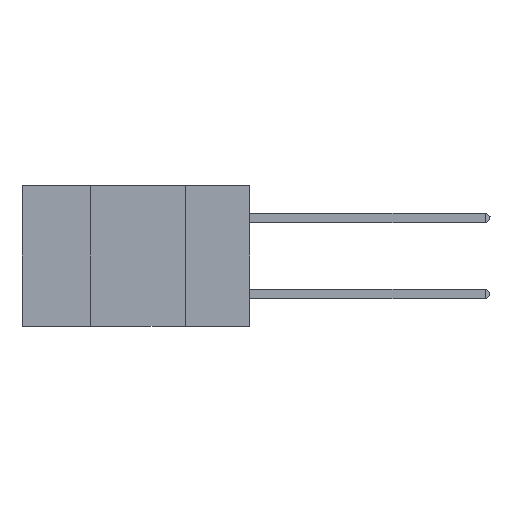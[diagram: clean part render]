
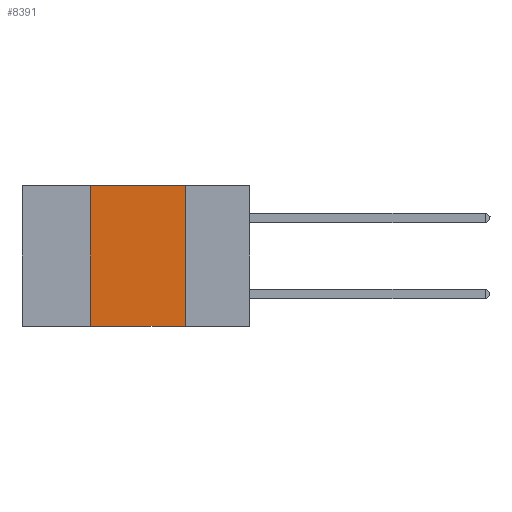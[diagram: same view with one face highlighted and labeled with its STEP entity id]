
A CAD part, left-side view. The second image highlights one B-rep face of the part: STEP entity #8391.
In plain terms, the highlighted planar face has unit normal (-1, 0, 0).
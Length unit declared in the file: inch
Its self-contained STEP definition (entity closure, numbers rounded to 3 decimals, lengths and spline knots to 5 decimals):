
#158 = CARTESIAN_POINT ( 'NONE',  ( 0., 0.42, 0. ) ) ;
#355 = VECTOR ( 'NONE', #10281, 39.37008 ) ;
#591 = EDGE_LOOP ( 'NONE', ( #8766, #2597, #5451, #9386 ) ) ;
#1286 = EDGE_CURVE ( 'NONE', #2280, #1753, #9003, .T. ) ;
#1416 = DIRECTION ( 'NONE',  ( 0., -1., 0. ) ) ;
#1703 = PLANE ( 'NONE',  #7467 ) ;
#1753 = VERTEX_POINT ( 'NONE', #158 ) ;
#2150 = EDGE_CURVE ( 'NONE', #5757, #7885, #3009, .T. ) ;
#2280 = VERTEX_POINT ( 'NONE', #3708 ) ;
#2571 = DIRECTION ( 'NONE',  ( 0., 0., -1. ) ) ;
#2597 = ORIENTED_EDGE ( 'NONE', *, *, #6865, .F. ) ;
#2881 = CARTESIAN_POINT ( 'NONE',  ( 0., 0.17, 0. ) ) ;
#3009 = LINE ( 'NONE', #8593, #3290 ) ;
#3290 = VECTOR ( 'NONE', #4409, 39.37008 ) ;
#3360 = CARTESIAN_POINT ( 'NONE',  ( 0., 0.6, 0. ) ) ;
#3565 = CARTESIAN_POINT ( 'NONE',  ( 0., 0.6, 0. ) ) ;
#3708 = CARTESIAN_POINT ( 'NONE',  ( 0., 0.42, -0.37 ) ) ;
#4179 = EDGE_CURVE ( 'NONE', #2280, #7885, #5869, .T. ) ;
#4409 = DIRECTION ( 'NONE',  ( 0., 0., -1. ) ) ;
#4703 = FACE_OUTER_BOUND ( 'NONE', #591, .T. ) ;
#5310 = VECTOR ( 'NONE', #1416, 39.37008 ) ;
#5451 = ORIENTED_EDGE ( 'NONE', *, *, #1286, .F. ) ;
#5757 = VERTEX_POINT ( 'NONE', #2881 ) ;
#5869 = LINE ( 'NONE', #6699, #9162 ) ;
#6699 = CARTESIAN_POINT ( 'NONE',  ( 0., 0.6, -0.37 ) ) ;
#6865 = EDGE_CURVE ( 'NONE', #1753, #5757, #11608, .T. ) ;
#7467 = AXIS2_PLACEMENT_3D ( 'NONE', #3565, #10190, #2571 ) ;
#7885 = VERTEX_POINT ( 'NONE', #8900 ) ;
#8391 = ADVANCED_FACE ( 'NONE', ( #4703 ), #1703, .F. ) ;
#8560 = DIRECTION ( 'NONE',  ( 0., -1., 0. ) ) ;
#8593 = CARTESIAN_POINT ( 'NONE',  ( 0., 0.17, 0. ) ) ;
#8766 = ORIENTED_EDGE ( 'NONE', *, *, #2150, .F. ) ;
#8900 = CARTESIAN_POINT ( 'NONE',  ( 0., 0.17, -0.37 ) ) ;
#9003 = LINE ( 'NONE', #9350, #355 ) ;
#9162 = VECTOR ( 'NONE', #8560, 39.37008 ) ;
#9350 = CARTESIAN_POINT ( 'NONE',  ( 0., 0.42, 0. ) ) ;
#9386 = ORIENTED_EDGE ( 'NONE', *, *, #4179, .T. ) ;
#10190 = DIRECTION ( 'NONE',  ( 1., 0., 0. ) ) ;
#10281 = DIRECTION ( 'NONE',  ( 0., 0., 1. ) ) ;
#11608 = LINE ( 'NONE', #3360, #5310 ) ;
